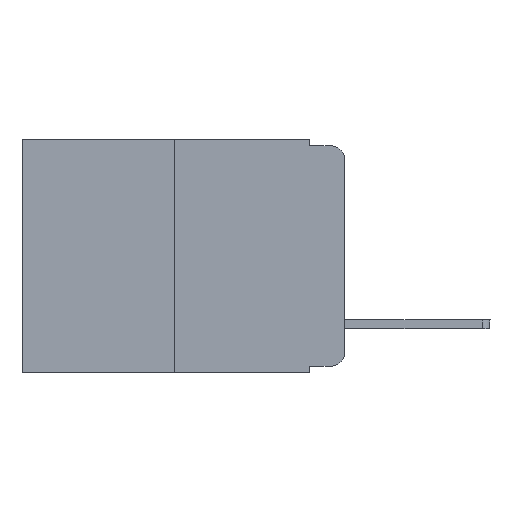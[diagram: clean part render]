
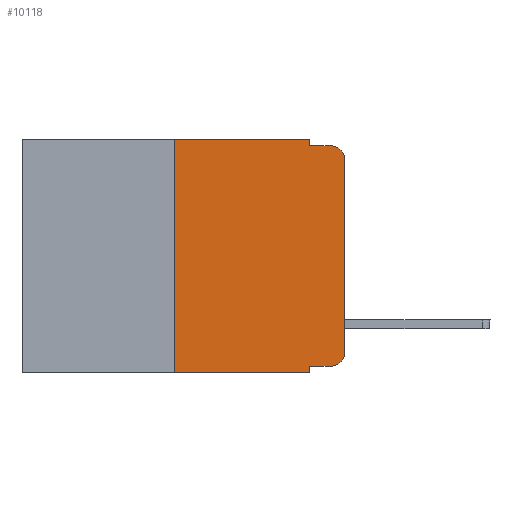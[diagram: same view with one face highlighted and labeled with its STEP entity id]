
A CAD part, left-side view. The second image highlights one B-rep face of the part: STEP entity #10118.
In plain terms, the highlighted planar face has unit normal (-1, 0, 0).
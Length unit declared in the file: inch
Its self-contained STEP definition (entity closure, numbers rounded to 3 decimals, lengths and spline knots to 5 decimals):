
#154 = EDGE_CURVE ( 'NONE', #11500, #8248, #7407, .T. ) ;
#265 = VECTOR ( 'NONE', #10437, 39.37008 ) ;
#286 = VERTEX_POINT ( 'NONE', #853 ) ;
#333 = DIRECTION ( 'NONE',  ( 0., 0., 1. ) ) ;
#340 = LINE ( 'NONE', #412, #4877 ) ;
#384 = VECTOR ( 'NONE', #12147, 39.37008 ) ;
#412 = CARTESIAN_POINT ( 'NONE',  ( 0., 0.051, 0. ) ) ;
#574 = DIRECTION ( 'NONE',  ( -1., 0., 0. ) ) ;
#591 = CARTESIAN_POINT ( 'NONE',  ( 0., 0.051, 0. ) ) ;
#853 = CARTESIAN_POINT ( 'NONE',  ( 0., 0., -0.03 ) ) ;
#928 = CIRCLE ( 'NONE', #7275, 0.02 ) ;
#948 = VERTEX_POINT ( 'NONE', #969 ) ;
#969 = CARTESIAN_POINT ( 'NONE',  ( 0., 0.25, 0. ) ) ;
#1003 = CARTESIAN_POINT ( 'NONE',  ( 0., 0.051, -0.333 ) ) ;
#1187 = VECTOR ( 'NONE', #333, 39.37008 ) ;
#1309 = PLANE ( 'NONE',  #3945 ) ;
#1379 = VERTEX_POINT ( 'NONE', #2691 ) ;
#1485 = DIRECTION ( 'NONE',  ( 0., 0., -1. ) ) ;
#1594 = CARTESIAN_POINT ( 'NONE',  ( 0., 0.02, -0.03 ) ) ;
#1631 = DIRECTION ( 'NONE',  ( 0., 0., -1. ) ) ;
#1722 = FACE_OUTER_BOUND ( 'NONE', #5579, .T. ) ;
#1730 = CARTESIAN_POINT ( 'NONE',  ( 0., 0.473, 0. ) ) ;
#2268 = DIRECTION ( 'NONE',  ( 0., 0., -1. ) ) ;
#2353 = ORIENTED_EDGE ( 'NONE', *, *, #7689, .F. ) ;
#2691 = CARTESIAN_POINT ( 'NONE',  ( 0., 0.051, -0.333 ) ) ;
#2763 = EDGE_CURVE ( 'NONE', #7587, #9898, #11719, .T. ) ;
#2889 = CARTESIAN_POINT ( 'NONE',  ( 0., 0.25, -0.343 ) ) ;
#2919 = CARTESIAN_POINT ( 'NONE',  ( 0., 0.051, -0.01 ) ) ;
#3611 = ORIENTED_EDGE ( 'NONE', *, *, #3630, .F. ) ;
#3630 = EDGE_CURVE ( 'NONE', #1379, #9898, #340, .T. ) ;
#3771 = EDGE_CURVE ( 'NONE', #286, #7055, #928, .T. ) ;
#3945 = AXIS2_PLACEMENT_3D ( 'NONE', #6935, #4085, #11739 ) ;
#3957 = ORIENTED_EDGE ( 'NONE', *, *, #3771, .T. ) ;
#4026 = CARTESIAN_POINT ( 'NONE',  ( 0., 0.02, -0.01 ) ) ;
#4043 = CARTESIAN_POINT ( 'NONE',  ( 0., 0., -0.313 ) ) ;
#4080 = VERTEX_POINT ( 'NONE', #9594 ) ;
#4085 = DIRECTION ( 'NONE',  ( 1., 0., 0. ) ) ;
#4495 = CARTESIAN_POINT ( 'NONE',  ( 0., 0., 0. ) ) ;
#4515 = LINE ( 'NONE', #1003, #265 ) ;
#4791 = CARTESIAN_POINT ( 'NONE',  ( 0., 0.051, -0.343 ) ) ;
#4841 = VERTEX_POINT ( 'NONE', #6206 ) ;
#4877 = VECTOR ( 'NONE', #2268, 39.37008 ) ;
#5153 = ORIENTED_EDGE ( 'NONE', *, *, #2763, .T. ) ;
#5274 = ORIENTED_EDGE ( 'NONE', *, *, #11328, .F. ) ;
#5579 = EDGE_LOOP ( 'NONE', ( #10895, #3957, #9023, #5274, #6746, #2353, #5153, #3611, #8774, #8743 ) ) ;
#5913 = CARTESIAN_POINT ( 'NONE',  ( 0., 0.25, 0. ) ) ;
#6206 = CARTESIAN_POINT ( 'NONE',  ( 0., 0.051, -0.01 ) ) ;
#6253 = EDGE_CURVE ( 'NONE', #4841, #7055, #10529, .T. ) ;
#6359 = CARTESIAN_POINT ( 'NONE',  ( 0., 0.02, -0.333 ) ) ;
#6746 = ORIENTED_EDGE ( 'NONE', *, *, #11844, .F. ) ;
#6769 = VECTOR ( 'NONE', #10543, 39.37008 ) ;
#6935 = CARTESIAN_POINT ( 'NONE',  ( 0., 0.473, 0. ) ) ;
#7055 = VERTEX_POINT ( 'NONE', #4026 ) ;
#7275 = AXIS2_PLACEMENT_3D ( 'NONE', #1594, #574, #1631 ) ;
#7407 = CIRCLE ( 'NONE', #10684, 0.02 ) ;
#7587 = VERTEX_POINT ( 'NONE', #2889 ) ;
#7689 = EDGE_CURVE ( 'NONE', #7587, #948, #9877, .T. ) ;
#8044 = LINE ( 'NONE', #1730, #11780 ) ;
#8248 = VERTEX_POINT ( 'NONE', #4043 ) ;
#8277 = VECTOR ( 'NONE', #1485, 39.37008 ) ;
#8743 = ORIENTED_EDGE ( 'NONE', *, *, #154, .T. ) ;
#8774 = ORIENTED_EDGE ( 'NONE', *, *, #9349, .T. ) ;
#9023 = ORIENTED_EDGE ( 'NONE', *, *, #6253, .F. ) ;
#9349 = EDGE_CURVE ( 'NONE', #1379, #11500, #4515, .T. ) ;
#9580 = CARTESIAN_POINT ( 'NONE',  ( 0., 0.02, -0.313 ) ) ;
#9594 = CARTESIAN_POINT ( 'NONE',  ( 0., 0.051, 0. ) ) ;
#9877 = LINE ( 'NONE', #5913, #1187 ) ;
#9898 = VERTEX_POINT ( 'NONE', #4791 ) ;
#9941 = LINE ( 'NONE', #4495, #384 ) ;
#10118 = ADVANCED_FACE ( 'NONE', ( #1722 ), #1309, .F. ) ;
#10398 = DIRECTION ( 'NONE',  ( 0., -1., 0. ) ) ;
#10416 = EDGE_CURVE ( 'NONE', #8248, #286, #9941, .T. ) ;
#10437 = DIRECTION ( 'NONE',  ( 0., -1., 0. ) ) ;
#10445 = DIRECTION ( 'NONE',  ( 0., 0., -1. ) ) ;
#10529 = LINE ( 'NONE', #2919, #6769 ) ;
#10543 = DIRECTION ( 'NONE',  ( 0., -1., 0. ) ) ;
#10579 = DIRECTION ( 'NONE',  ( -1., 0., 0. ) ) ;
#10684 = AXIS2_PLACEMENT_3D ( 'NONE', #9580, #10579, #10445 ) ;
#10850 = VECTOR ( 'NONE', #10398, 39.37008 ) ;
#10854 = LINE ( 'NONE', #591, #8277 ) ;
#10895 = ORIENTED_EDGE ( 'NONE', *, *, #10416, .T. ) ;
#11074 = DIRECTION ( 'NONE',  ( 0., -1., 0. ) ) ;
#11266 = CARTESIAN_POINT ( 'NONE',  ( 0., 0.473, -0.343 ) ) ;
#11328 = EDGE_CURVE ( 'NONE', #4080, #4841, #10854, .T. ) ;
#11500 = VERTEX_POINT ( 'NONE', #6359 ) ;
#11719 = LINE ( 'NONE', #11266, #10850 ) ;
#11739 = DIRECTION ( 'NONE',  ( 0., 0., -1. ) ) ;
#11780 = VECTOR ( 'NONE', #11074, 39.37008 ) ;
#11844 = EDGE_CURVE ( 'NONE', #948, #4080, #8044, .T. ) ;
#12147 = DIRECTION ( 'NONE',  ( 0., 0., 1. ) ) ;
